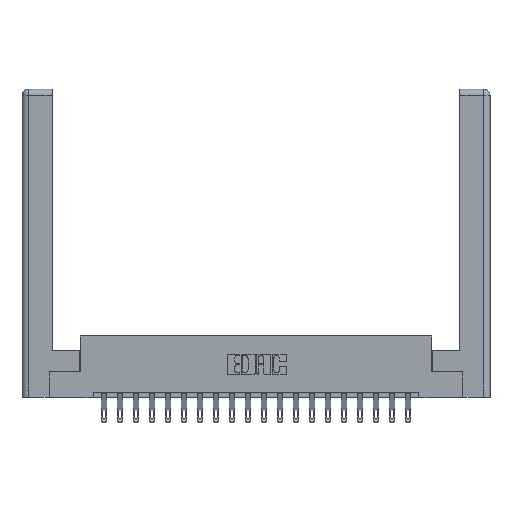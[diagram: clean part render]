
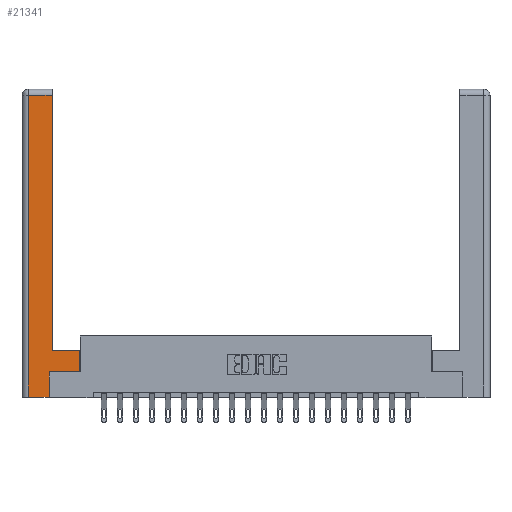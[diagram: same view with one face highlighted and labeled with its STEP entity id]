
A CAD part, top view. The second image highlights one B-rep face of the part: STEP entity #21341.
In plain terms, the highlighted planar face has unit normal (0, 0, 1).
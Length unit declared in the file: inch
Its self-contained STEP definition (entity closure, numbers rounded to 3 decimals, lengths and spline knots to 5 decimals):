
#70 = VECTOR ( 'NONE', #19953, 39.37008 ) ;
#1018 = EDGE_CURVE ( 'NONE', #5205, #1270, #20661, .T. ) ;
#1188 = CARTESIAN_POINT ( 'NONE',  ( 0.265, 0.245, 0. ) ) ;
#1270 = VERTEX_POINT ( 'NONE', #19669 ) ;
#1386 = EDGE_CURVE ( 'NONE', #16229, #11102, #7041, .T. ) ;
#1675 = LINE ( 'NONE', #4323, #10701 ) ;
#1893 = LINE ( 'NONE', #2606, #13505 ) ;
#1913 = FACE_OUTER_BOUND ( 'NONE', #9319, .T. ) ;
#2057 = EDGE_CURVE ( 'NONE', #5986, #9958, #16553, .T. ) ;
#2114 = AXIS2_PLACEMENT_3D ( 'NONE', #2220, #20449, #13907 ) ;
#2220 = CARTESIAN_POINT ( 'NONE',  ( 0., 0., 0. ) ) ;
#2606 = CARTESIAN_POINT ( 'NONE',  ( 0.0615, 0., 0. ) ) ;
#3139 = VECTOR ( 'NONE', #20545, 39.37008 ) ;
#3527 = VECTOR ( 'NONE', #6246, 39.37008 ) ;
#3963 = ORIENTED_EDGE ( 'NONE', *, *, #18089, .T. ) ;
#4119 = CARTESIAN_POINT ( 'NONE',  ( 0.0615, 2.94, 0. ) ) ;
#4323 = CARTESIAN_POINT ( 'NONE',  ( 0.565, 0.45, 0. ) ) ;
#4768 = CARTESIAN_POINT ( 'NONE',  ( 0.265, 0., 0. ) ) ;
#4865 = CARTESIAN_POINT ( 'NONE',  ( 0.295, 2.94, 0. ) ) ;
#5205 = VERTEX_POINT ( 'NONE', #4865 ) ;
#5528 = CARTESIAN_POINT ( 'NONE',  ( 0.0615, 0., 0. ) ) ;
#5986 = VERTEX_POINT ( 'NONE', #6802 ) ;
#6142 = EDGE_CURVE ( 'NONE', #9958, #16860, #1675, .T. ) ;
#6246 = DIRECTION ( 'NONE',  ( 0., 1., 0. ) ) ;
#6802 = CARTESIAN_POINT ( 'NONE',  ( 0.265, 0.245, 0. ) ) ;
#6827 = CARTESIAN_POINT ( 'NONE',  ( 0.265, 0., 0. ) ) ;
#7041 = LINE ( 'NONE', #4768, #70 ) ;
#7567 = DIRECTION ( 'NONE',  ( -1., 0., 0. ) ) ;
#8155 = LINE ( 'NONE', #1188, #3527 ) ;
#8169 = VECTOR ( 'NONE', #7567, 39.37008 ) ;
#9104 = LINE ( 'NONE', #10763, #14776 ) ;
#9319 = EDGE_LOOP ( 'NONE', ( #3963, #20464, #15339, #20709, #9712, #16685, #14312, #20622 ) ) ;
#9361 = DIRECTION ( 'NONE',  ( 0., 1., 0. ) ) ;
#9712 = ORIENTED_EDGE ( 'NONE', *, *, #14783, .T. ) ;
#9958 = VERTEX_POINT ( 'NONE', #11969 ) ;
#9999 = EDGE_CURVE ( 'NONE', #16860, #13166, #19769, .T. ) ;
#10451 = CARTESIAN_POINT ( 'NONE',  ( 0.295, 0.45, 0. ) ) ;
#10701 = VECTOR ( 'NONE', #9361, 39.37008 ) ;
#10763 = CARTESIAN_POINT ( 'NONE',  ( 0.295, 3., 0. ) ) ;
#11102 = VERTEX_POINT ( 'NONE', #6827 ) ;
#11561 = CARTESIAN_POINT ( 'NONE',  ( 0.565, 0.245, 0. ) ) ;
#11969 = CARTESIAN_POINT ( 'NONE',  ( 0.565, 0.245, 0. ) ) ;
#12540 = EDGE_CURVE ( 'NONE', #1270, #16229, #1893, .T. ) ;
#13166 = VERTEX_POINT ( 'NONE', #10451 ) ;
#13505 = VECTOR ( 'NONE', #17240, 39.37008 ) ;
#13516 = CARTESIAN_POINT ( 'NONE',  ( 0.565, 0.45, 0. ) ) ;
#13907 = DIRECTION ( 'NONE',  ( -1., 0., 0. ) ) ;
#14312 = ORIENTED_EDGE ( 'NONE', *, *, #6142, .T. ) ;
#14776 = VECTOR ( 'NONE', #15448, 39.37008 ) ;
#14783 = EDGE_CURVE ( 'NONE', #11102, #5986, #8155, .T. ) ;
#15339 = ORIENTED_EDGE ( 'NONE', *, *, #12540, .T. ) ;
#15448 = DIRECTION ( 'NONE',  ( 0., 1., 0. ) ) ;
#15634 = CARTESIAN_POINT ( 'NONE',  ( 0.295, 0.45, 0. ) ) ;
#16229 = VERTEX_POINT ( 'NONE', #5528 ) ;
#16553 = LINE ( 'NONE', #11561, #20403 ) ;
#16685 = ORIENTED_EDGE ( 'NONE', *, *, #2057, .T. ) ;
#16860 = VERTEX_POINT ( 'NONE', #13516 ) ;
#17240 = DIRECTION ( 'NONE',  ( 0., -1., 0. ) ) ;
#18089 = EDGE_CURVE ( 'NONE', #13166, #5205, #9104, .T. ) ;
#18785 = PLANE ( 'NONE',  #2114 ) ;
#19669 = CARTESIAN_POINT ( 'NONE',  ( 0.0615, 2.94, 0. ) ) ;
#19769 = LINE ( 'NONE', #15634, #8169 ) ;
#19829 = DIRECTION ( 'NONE',  ( 1., 0., 0. ) ) ;
#19953 = DIRECTION ( 'NONE',  ( 1., 0., 0. ) ) ;
#20403 = VECTOR ( 'NONE', #19829, 39.37008 ) ;
#20449 = DIRECTION ( 'NONE',  ( 0., 0., -1. ) ) ;
#20464 = ORIENTED_EDGE ( 'NONE', *, *, #1018, .T. ) ;
#20545 = DIRECTION ( 'NONE',  ( -1., 0., 0. ) ) ;
#20622 = ORIENTED_EDGE ( 'NONE', *, *, #9999, .T. ) ;
#20661 = LINE ( 'NONE', #4119, #3139 ) ;
#20709 = ORIENTED_EDGE ( 'NONE', *, *, #1386, .T. ) ;
#21341 = ADVANCED_FACE ( 'NONE', ( #1913 ), #18785, .F. ) ;
